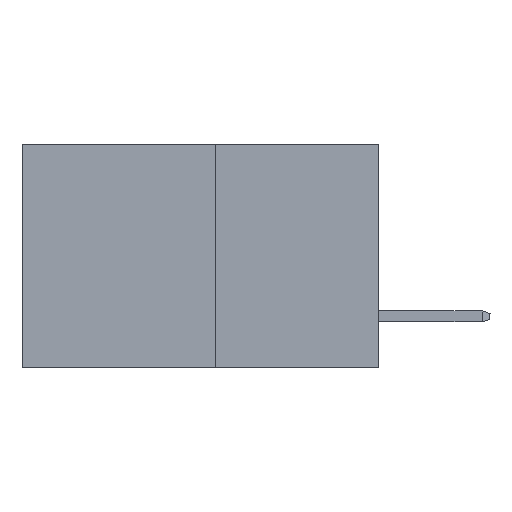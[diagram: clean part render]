
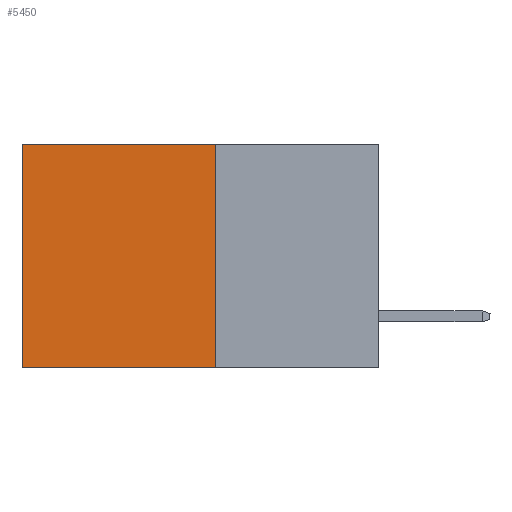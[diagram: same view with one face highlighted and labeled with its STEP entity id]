
A CAD part, left-side view. The second image highlights one B-rep face of the part: STEP entity #5450.
In plain terms, the highlighted planar face has unit normal (-1, 0, 0).
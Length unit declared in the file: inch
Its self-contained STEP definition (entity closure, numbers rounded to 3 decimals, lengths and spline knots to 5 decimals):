
#2052 = LINE ( 'NONE', #11753, #12984 ) ;
#2417 = ORIENTED_EDGE ( 'NONE', *, *, #2880, .T. ) ;
#2880 = EDGE_CURVE ( 'NONE', #14743, #21878, #2052, .T. ) ;
#3693 = ORIENTED_EDGE ( 'NONE', *, *, #20794, .F. ) ;
#4908 = VECTOR ( 'NONE', #13311, 39.37008 ) ;
#5450 = ADVANCED_FACE ( 'NONE', ( #14613 ), #23572, .F. ) ;
#5931 = DIRECTION ( 'NONE',  ( 0., 0., -1. ) ) ;
#6055 = VERTEX_POINT ( 'NONE', #26540 ) ;
#6120 = DIRECTION ( 'NONE',  ( 0., 1., 0. ) ) ;
#7331 = LINE ( 'NONE', #10207, #12430 ) ;
#8443 = CARTESIAN_POINT ( 'NONE',  ( 0.277, 0.27, 0. ) ) ;
#8517 = EDGE_LOOP ( 'NONE', ( #25632, #21415, #3693, #2417 ) ) ;
#8954 = CARTESIAN_POINT ( 'NONE',  ( 0.277, 0.59, -0.37 ) ) ;
#10207 = CARTESIAN_POINT ( 'NONE',  ( 0.277, 0.27, -0.37 ) ) ;
#10977 = DIRECTION ( 'NONE',  ( 0., 1., 0. ) ) ;
#11753 = CARTESIAN_POINT ( 'NONE',  ( 0.277, 0.27, 0. ) ) ;
#12430 = VECTOR ( 'NONE', #5931, 39.37008 ) ;
#12984 = VECTOR ( 'NONE', #10977, 39.37008 ) ;
#13311 = DIRECTION ( 'NONE',  ( 0., 0., -1. ) ) ;
#13584 = AXIS2_PLACEMENT_3D ( 'NONE', #20347, #27203, #27162 ) ;
#14034 = EDGE_CURVE ( 'NONE', #6055, #27330, #21859, .T. ) ;
#14613 = FACE_OUTER_BOUND ( 'NONE', #8517, .T. ) ;
#14743 = VERTEX_POINT ( 'NONE', #8443 ) ;
#19015 = CARTESIAN_POINT ( 'NONE',  ( 0.277, 0.59, -0.37 ) ) ;
#20347 = CARTESIAN_POINT ( 'NONE',  ( 0.277, 0.27, -0.37 ) ) ;
#20794 = EDGE_CURVE ( 'NONE', #14743, #6055, #7331, .T. ) ;
#21070 = EDGE_CURVE ( 'NONE', #21878, #27330, #28307, .T. ) ;
#21415 = ORIENTED_EDGE ( 'NONE', *, *, #14034, .F. ) ;
#21859 = LINE ( 'NONE', #23665, #25703 ) ;
#21878 = VERTEX_POINT ( 'NONE', #23488 ) ;
#23488 = CARTESIAN_POINT ( 'NONE',  ( 0.277, 0.59, 0. ) ) ;
#23572 = PLANE ( 'NONE',  #13584 ) ;
#23665 = CARTESIAN_POINT ( 'NONE',  ( 0.277, 0.27, -0.37 ) ) ;
#25632 = ORIENTED_EDGE ( 'NONE', *, *, #21070, .T. ) ;
#25703 = VECTOR ( 'NONE', #6120, 39.37008 ) ;
#26540 = CARTESIAN_POINT ( 'NONE',  ( 0.277, 0.27, -0.37 ) ) ;
#27162 = DIRECTION ( 'NONE',  ( 0., 0., -1. ) ) ;
#27203 = DIRECTION ( 'NONE',  ( 1., 0., 0. ) ) ;
#27330 = VERTEX_POINT ( 'NONE', #19015 ) ;
#28307 = LINE ( 'NONE', #8954, #4908 ) ;
